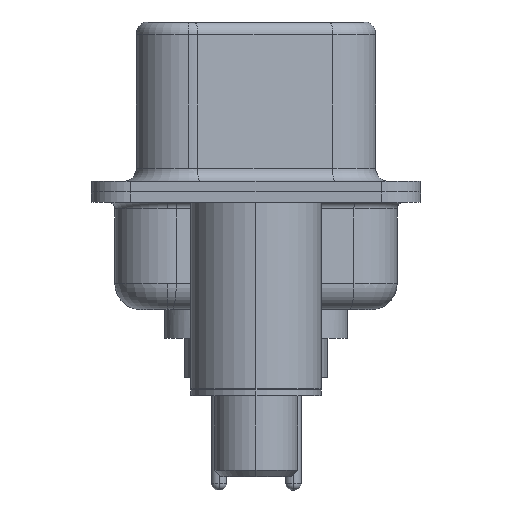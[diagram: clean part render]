
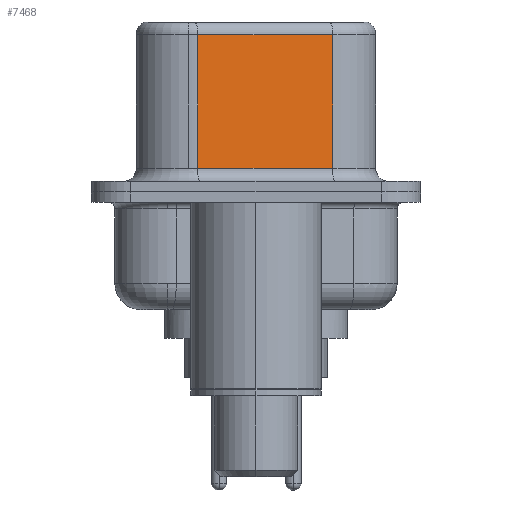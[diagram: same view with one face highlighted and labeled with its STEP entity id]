
A CAD part, left-side view. The second image highlights one B-rep face of the part: STEP entity #7468.
In plain terms, the highlighted planar face has unit normal (-0.985, -0.174, 0).
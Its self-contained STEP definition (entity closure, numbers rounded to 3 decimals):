
#583 = LINE ( 'NONE', #21043, #7483 ) ;
#798 = ORIENTED_EDGE ( 'NONE', *, *, #12391, .T. ) ;
#803 = DIRECTION ( 'NONE',  ( 0.174, -0.985, 0. ) ) ;
#962 = CARTESIAN_POINT ( 'NONE',  ( 3.675, 2.233, 0.9 ) ) ;
#1119 = LINE ( 'NONE', #4880, #4582 ) ;
#3459 = CARTESIAN_POINT ( 'NONE',  ( 3.675, 2.233, 6.52 ) ) ;
#3512 = CARTESIAN_POINT ( 'NONE',  ( 4.585, -2.927, 6.02 ) ) ;
#3723 = EDGE_CURVE ( 'NONE', #20916, #5335, #14441, .T. ) ;
#4045 = CARTESIAN_POINT ( 'NONE',  ( 4.585, -2.927, 0.9 ) ) ;
#4582 = VECTOR ( 'NONE', #18063, 1000. ) ;
#4880 = CARTESIAN_POINT ( 'NONE',  ( 4.585, -2.927, 6.02 ) ) ;
#5335 = VERTEX_POINT ( 'NONE', #962 ) ;
#5431 = AXIS2_PLACEMENT_3D ( 'NONE', #13380, #20742, #20592 ) ;
#6081 = EDGE_CURVE ( 'NONE', #5335, #8753, #583, .T. ) ;
#7020 = ORIENTED_EDGE ( 'NONE', *, *, #3723, .T. ) ;
#7468 = ADVANCED_FACE ( 'NONE', ( #12835 ), #7653, .F. ) ;
#7483 = VECTOR ( 'NONE', #803, 1000. ) ;
#7653 = PLANE ( 'NONE',  #5431 ) ;
#8753 = VERTEX_POINT ( 'NONE', #4045 ) ;
#11595 = EDGE_LOOP ( 'NONE', ( #12417, #798, #7020, #12177 ) ) ;
#12177 = ORIENTED_EDGE ( 'NONE', *, *, #6081, .T. ) ;
#12391 = EDGE_CURVE ( 'NONE', #12478, #20916, #1119, .T. ) ;
#12417 = ORIENTED_EDGE ( 'NONE', *, *, #20824, .F. ) ;
#12431 = VECTOR ( 'NONE', #21930, 1000. ) ;
#12478 = VERTEX_POINT ( 'NONE', #3512 ) ;
#12835 = FACE_OUTER_BOUND ( 'NONE', #11595, .T. ) ;
#13380 = CARTESIAN_POINT ( 'NONE',  ( 4.585, -2.927, 6.52 ) ) ;
#13540 = VECTOR ( 'NONE', #23333, 1000. ) ;
#14441 = LINE ( 'NONE', #3459, #13540 ) ;
#17292 = LINE ( 'NONE', #21695, #12431 ) ;
#18063 = DIRECTION ( 'NONE',  ( -0.174, 0.985, 0. ) ) ;
#20337 = CARTESIAN_POINT ( 'NONE',  ( 3.675, 2.233, 6.02 ) ) ;
#20592 = DIRECTION ( 'NONE',  ( -0.174, 0.985, 0. ) ) ;
#20742 = DIRECTION ( 'NONE',  ( 0.985, 0.174, 0. ) ) ;
#20824 = EDGE_CURVE ( 'NONE', #12478, #8753, #17292, .T. ) ;
#20916 = VERTEX_POINT ( 'NONE', #20337 ) ;
#21043 = CARTESIAN_POINT ( 'NONE',  ( 4.585, -2.927, 0.9 ) ) ;
#21695 = CARTESIAN_POINT ( 'NONE',  ( 4.585, -2.927, 6.52 ) ) ;
#21930 = DIRECTION ( 'NONE',  ( 0., 0., -1. ) ) ;
#23333 = DIRECTION ( 'NONE',  ( 0., 0., -1. ) ) ;
